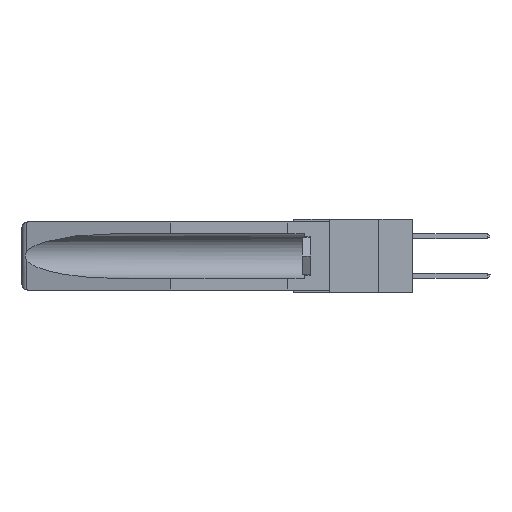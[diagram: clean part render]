
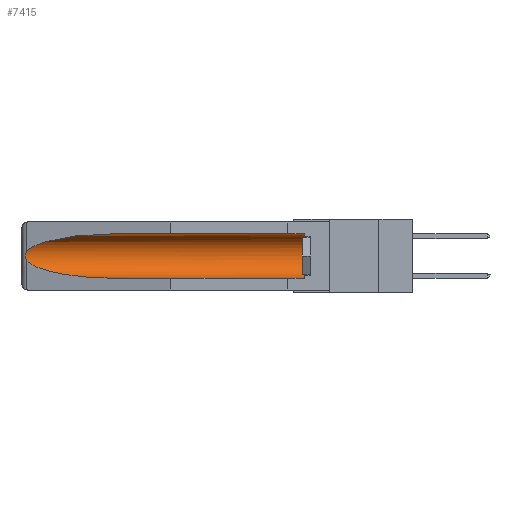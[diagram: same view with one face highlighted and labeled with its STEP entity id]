
A CAD part, left-side view. The second image highlights one B-rep face of the part: STEP entity #7415.
In plain terms, the highlighted cylindrical face has radius 2.857 mm (diameter 5.715 mm), a partial arc.
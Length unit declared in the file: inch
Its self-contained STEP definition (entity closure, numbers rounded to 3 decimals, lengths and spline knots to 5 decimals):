
#12 = EDGE_CURVE ( 'NONE', #541, #29036, #12745, .T. ) ;
#405 = AXIS2_PLACEMENT_3D ( 'NONE', #11521, #26969, #4377 ) ;
#541 = VERTEX_POINT ( 'NONE', #28682 ) ;
#641 = CARTESIAN_POINT ( 'NONE',  ( 0.2675, 1.53308, -0.17534 ) ) ;
#1020 = LINE ( 'NONE', #27626, #21902 ) ;
#1991 = CARTESIAN_POINT ( 'NONE',  ( 0.21114, 1.30732, -0.284 ) ) ;
#2411 = AXIS2_PLACEMENT_3D ( 'NONE', #3484, #28478, #26148 ) ;
#3142 = ORIENTED_EDGE ( 'NONE', *, *, #12, .T. ) ;
#3484 = CARTESIAN_POINT ( 'NONE',  ( 0.155, 0.126, -0.1715 ) ) ;
#3802 = CARTESIAN_POINT ( 'NONE',  ( 0.25451, 1.48313, -0.09465 ) ) ;
#4377 = DIRECTION ( 'NONE',  ( 0., 0., 1. ) ) ;
#4757 = CARTESIAN_POINT ( 'NONE',  ( 0.155, 0.126, -0.284 ) ) ;
#5233 = EDGE_CURVE ( 'NONE', #20280, #28189, #5476, .T. ) ;
#5476 = CIRCLE ( 'NONE', #2411, 0.1125 ) ;
#7024 = EDGE_CURVE ( 'NONE', #20280, #18297, #20927, .T. ) ;
#7083 = CYLINDRICAL_SURFACE ( 'NONE', #405, 0.1125 ) ;
#7415 = ADVANCED_FACE ( 'NONE', ( #25858 ), #7083, .F. ) ;
#8552 = EDGE_CURVE ( 'NONE', #9797, #541, #15413, .T. ) ;
#8912 = CARTESIAN_POINT ( 'NONE',  ( 0.155, 0.126, -0.059 ) ) ;
#8977 = ORIENTED_EDGE ( 'NONE', *, *, #18782, .T. ) ;
#9750 = CARTESIAN_POINT ( 'NONE',  ( 0.2675, 1.53308, -0.16763 ) ) ;
#9797 = VERTEX_POINT ( 'NONE', #11744 ) ;
#11521 = CARTESIAN_POINT ( 'NONE',  ( 0.155, -0.30754, -0.1715 ) ) ;
#11744 = CARTESIAN_POINT ( 'NONE',  ( 0.155, 1.07973, -0.059 ) ) ;
#12745 = B_SPLINE_CURVE_WITH_KNOTS ( 'NONE', 3,
 ( #25758, #25466, #14211, #21000, #9750, #641, #27978, #16493, #23560, #21314 ),
 .UNSPECIFIED., .F., .F.,
 ( 4, 2, 2, 2, 4 ),
 ( 0., 0.00029, 0.00058, 0.00087, 0.00117 ),
 .UNSPECIFIED. ) ;
#12990 = ORIENTED_EDGE ( 'NONE', *, *, #5233, .T. ) ;
#13373 = CARTESIAN_POINT ( 'NONE',  ( 0.155, -0.30754, -0.284 ) ) ;
#13866 = VECTOR ( 'NONE', #15752, 39.37008 ) ;
#14062 = DIRECTION ( 'NONE',  ( 0., 1., 0. ) ) ;
#14211 = CARTESIAN_POINT ( 'NONE',  ( 0.26654, 1.53092, -0.15636 ) ) ;
#15113 = EDGE_CURVE ( 'NONE', #28189, #9797, #1020, .T. ) ;
#15413 =( BOUNDED_CURVE ( )  B_SPLINE_CURVE ( 3, ( #19243, #23606, #3802, #28625 ),
 .UNSPECIFIED., .F., .F. ) 
 B_SPLINE_CURVE_WITH_KNOTS ( ( 4, 4 ),
 ( 4.71239, 6.08839 ),
 .UNSPECIFIED. ) 
 CURVE ( )  GEOMETRIC_REPRESENTATION_ITEM ( )  RATIONAL_B_SPLINE_CURVE ( ( 1., 0.848, 0.848, 1. ) ) 
 REPRESENTATION_ITEM ( '' )  );
#15752 = DIRECTION ( 'NONE',  ( 0., 1., 0. ) ) ;
#16392 = ORIENTED_EDGE ( 'NONE', *, *, #15113, .T. ) ;
#16493 = CARTESIAN_POINT ( 'NONE',  ( 0.26655, 1.53094, -0.18657 ) ) ;
#16885 =( BOUNDED_CURVE ( )  B_SPLINE_CURVE ( 3, ( #17716, #29159, #1991, #22472 ),
 .UNSPECIFIED., .F., .F. ) 
 B_SPLINE_CURVE_WITH_KNOTS ( ( 4, 4 ),
 ( 0.1948, 1.5708 ),
 .UNSPECIFIED. ) 
 CURVE ( )  GEOMETRIC_REPRESENTATION_ITEM ( )  RATIONAL_B_SPLINE_CURVE ( ( 1., 0.848, 0.848, 1. ) ) 
 REPRESENTATION_ITEM ( '' )  );
#17716 = CARTESIAN_POINT ( 'NONE',  ( 0.26537, 1.52718, -0.19328 ) ) ;
#18297 = VERTEX_POINT ( 'NONE', #27557 ) ;
#18782 = EDGE_CURVE ( 'NONE', #29036, #18297, #16885, .T. ) ;
#19243 = CARTESIAN_POINT ( 'NONE',  ( 0.155, 1.07973, -0.059 ) ) ;
#20280 = VERTEX_POINT ( 'NONE', #4757 ) ;
#20735 = ORIENTED_EDGE ( 'NONE', *, *, #7024, .F. ) ;
#20927 = LINE ( 'NONE', #13373, #13866 ) ;
#21000 = CARTESIAN_POINT ( 'NONE',  ( 0.2673, 1.5327, -0.16383 ) ) ;
#21314 = CARTESIAN_POINT ( 'NONE',  ( 0.26537, 1.52718, -0.19328 ) ) ;
#21902 = VECTOR ( 'NONE', #14062, 39.37008 ) ;
#22472 = CARTESIAN_POINT ( 'NONE',  ( 0.155, 1.07973, -0.284 ) ) ;
#23152 = ORIENTED_EDGE ( 'NONE', *, *, #8552, .T. ) ;
#23560 = CARTESIAN_POINT ( 'NONE',  ( 0.26597, 1.5296, -0.19026 ) ) ;
#23606 = CARTESIAN_POINT ( 'NONE',  ( 0.21114, 1.30732, -0.059 ) ) ;
#23659 = CARTESIAN_POINT ( 'NONE',  ( 0.26537, 1.52718, -0.19328 ) ) ;
#25466 = CARTESIAN_POINT ( 'NONE',  ( 0.26597, 1.52961, -0.15275 ) ) ;
#25734 = EDGE_LOOP ( 'NONE', ( #23152, #3142, #8977, #20735, #12990, #16392 ) ) ;
#25758 = CARTESIAN_POINT ( 'NONE',  ( 0.26537, 1.52718, -0.14972 ) ) ;
#25858 = FACE_OUTER_BOUND ( 'NONE', #25734, .T. ) ;
#26148 = DIRECTION ( 'NONE',  ( 0., 0., 1. ) ) ;
#26969 = DIRECTION ( 'NONE',  ( 0., 1., 0. ) ) ;
#27557 = CARTESIAN_POINT ( 'NONE',  ( 0.155, 1.07973, -0.284 ) ) ;
#27626 = CARTESIAN_POINT ( 'NONE',  ( 0.155, -0.30754, -0.059 ) ) ;
#27978 = CARTESIAN_POINT ( 'NONE',  ( 0.2673, 1.53269, -0.17917 ) ) ;
#28189 = VERTEX_POINT ( 'NONE', #8912 ) ;
#28478 = DIRECTION ( 'NONE',  ( 0., -1., 0. ) ) ;
#28625 = CARTESIAN_POINT ( 'NONE',  ( 0.26537, 1.52718, -0.14972 ) ) ;
#28682 = CARTESIAN_POINT ( 'NONE',  ( 0.26537, 1.52718, -0.14972 ) ) ;
#29036 = VERTEX_POINT ( 'NONE', #23659 ) ;
#29159 = CARTESIAN_POINT ( 'NONE',  ( 0.25451, 1.48313, -0.24835 ) ) ;
